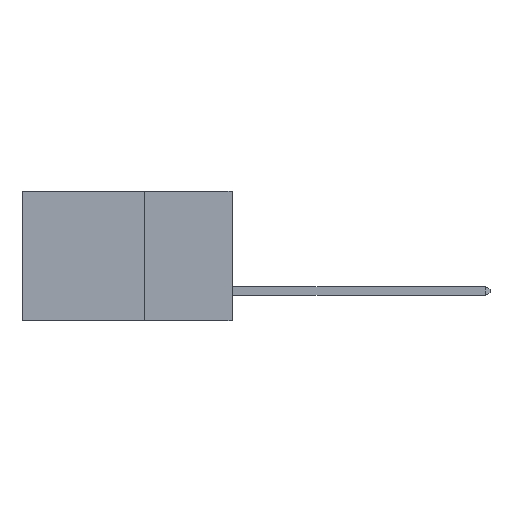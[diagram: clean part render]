
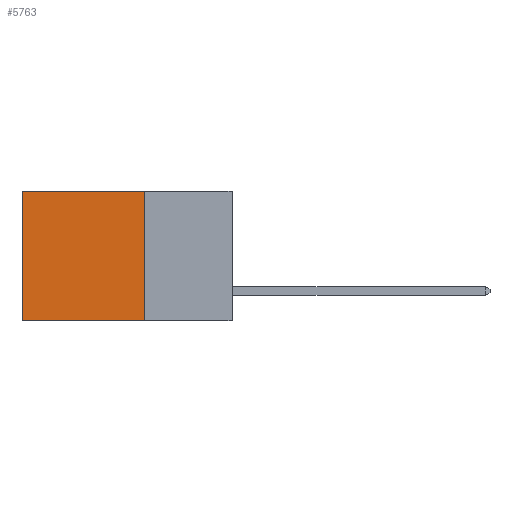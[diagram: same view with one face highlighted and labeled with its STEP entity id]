
A CAD part, left-side view. The second image highlights one B-rep face of the part: STEP entity #5763.
In plain terms, the highlighted planar face has unit normal (-1, 0, 0).
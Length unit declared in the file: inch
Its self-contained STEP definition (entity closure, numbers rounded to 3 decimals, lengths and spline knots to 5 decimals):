
#1211 = EDGE_CURVE ( 'NONE', #10853, #11676, #11740, .T. ) ;
#1247 = CARTESIAN_POINT ( 'NONE',  ( 0.2875, 0.25, 0. ) ) ;
#1574 = CARTESIAN_POINT ( 'NONE',  ( 0.2875, 0.6, -0.37 ) ) ;
#2025 = ORIENTED_EDGE ( 'NONE', *, *, #11970, .F. ) ;
#3518 = CARTESIAN_POINT ( 'NONE',  ( 0.2875, 0.25, 0. ) ) ;
#3953 = EDGE_LOOP ( 'NONE', ( #10855, #16536, #2025, #7143 ) ) ;
#4748 = DIRECTION ( 'NONE',  ( 0., 1., 0. ) ) ;
#5558 = DIRECTION ( 'NONE',  ( 0., 0., -1. ) ) ;
#5678 = CARTESIAN_POINT ( 'NONE',  ( 0.2875, 0.6, 0. ) ) ;
#5763 = ADVANCED_FACE ( 'NONE', ( #15281 ), #6712, .F. ) ;
#6193 = AXIS2_PLACEMENT_3D ( 'NONE', #6854, #6221, #5558 ) ;
#6221 = DIRECTION ( 'NONE',  ( 1., 0., 0. ) ) ;
#6675 = CARTESIAN_POINT ( 'NONE',  ( 0.2875, 0.25, -0.37 ) ) ;
#6712 = PLANE ( 'NONE',  #6193 ) ;
#6854 = CARTESIAN_POINT ( 'NONE',  ( 0.2875, 0.25, 0. ) ) ;
#7143 = ORIENTED_EDGE ( 'NONE', *, *, #1211, .T. ) ;
#7363 = CARTESIAN_POINT ( 'NONE',  ( 0.2875, 0.25, 0. ) ) ;
#8438 = VECTOR ( 'NONE', #4748, 39.37008 ) ;
#8855 = LINE ( 'NONE', #12769, #8438 ) ;
#9077 = VERTEX_POINT ( 'NONE', #6675 ) ;
#9704 = LINE ( 'NONE', #5678, #16631 ) ;
#10773 = EDGE_CURVE ( 'NONE', #9077, #11836, #8855, .T. ) ;
#10853 = VERTEX_POINT ( 'NONE', #3518 ) ;
#10855 = ORIENTED_EDGE ( 'NONE', *, *, #15316, .T. ) ;
#11003 = DIRECTION ( 'NONE',  ( 0., 0., -1. ) ) ;
#11333 = VECTOR ( 'NONE', #17295, 39.37008 ) ;
#11355 = DIRECTION ( 'NONE',  ( 0., 0., -1. ) ) ;
#11676 = VERTEX_POINT ( 'NONE', #16039 ) ;
#11740 = LINE ( 'NONE', #1247, #11333 ) ;
#11836 = VERTEX_POINT ( 'NONE', #1574 ) ;
#11970 = EDGE_CURVE ( 'NONE', #10853, #9077, #13799, .T. ) ;
#12769 = CARTESIAN_POINT ( 'NONE',  ( 0.2875, 0.25, -0.37 ) ) ;
#13397 = VECTOR ( 'NONE', #11355, 39.37008 ) ;
#13799 = LINE ( 'NONE', #7363, #13397 ) ;
#15281 = FACE_OUTER_BOUND ( 'NONE', #3953, .T. ) ;
#15316 = EDGE_CURVE ( 'NONE', #11676, #11836, #9704, .T. ) ;
#16039 = CARTESIAN_POINT ( 'NONE',  ( 0.2875, 0.6, 0. ) ) ;
#16536 = ORIENTED_EDGE ( 'NONE', *, *, #10773, .F. ) ;
#16631 = VECTOR ( 'NONE', #11003, 39.37008 ) ;
#17295 = DIRECTION ( 'NONE',  ( 0., 1., 0. ) ) ;
